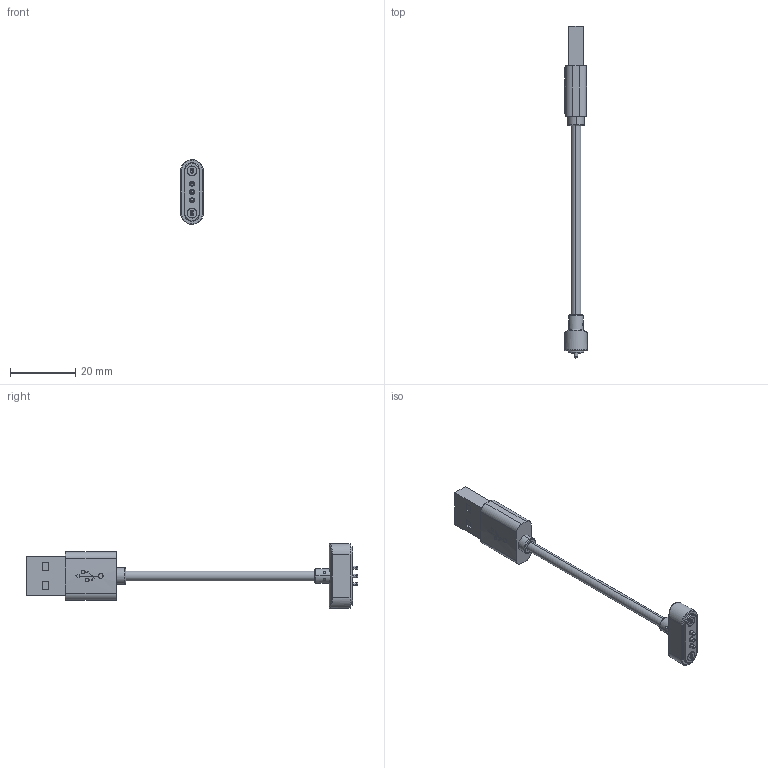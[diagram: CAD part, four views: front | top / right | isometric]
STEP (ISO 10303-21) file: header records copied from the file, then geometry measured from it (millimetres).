
FILE_DESCRIPTION (( 'STEP AP203' ), '1' );
FILE_NAME ('687-D0322A110100.STEP', '2023-02-14T13:29:03', ( 'Magnum' ), ( '' ), 'SwSTEP 2.0', 'SolidWorks 2020', '' );
FILE_SCHEMA (( 'CONFIG_CONTROL_DESIGN' ));
Length unit declared in the file: millimetre
Products named in the file (1): 687-D0322A110100
Bounding box: 6.9 x 102.05 x 19.9 mm (x, y, z)
Volume: 3214.5 mm3; surface area: 2762.7 mm2
Topology: 2 solids, 4 shells, 199 faces, 486 edges, 311 vertices
Faces by surface type: plane 74, cylinder 63, bspline 34, torus 14, cone 8, sphere 6
Entity records: 8427 total; most frequent: CARTESIAN_POINT 3892, ORIENTED_EDGE 948, DIRECTION 844, EDGE_CURVE 474, VERTEX_POINT 305, AXIS2_PLACEMENT_3D 299, LINE 246, VECTOR 246
